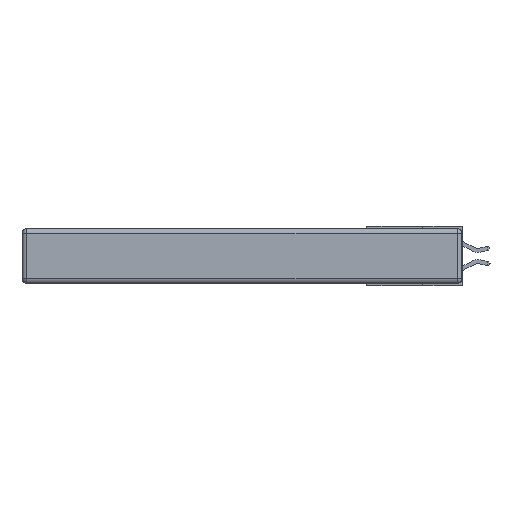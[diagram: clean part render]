
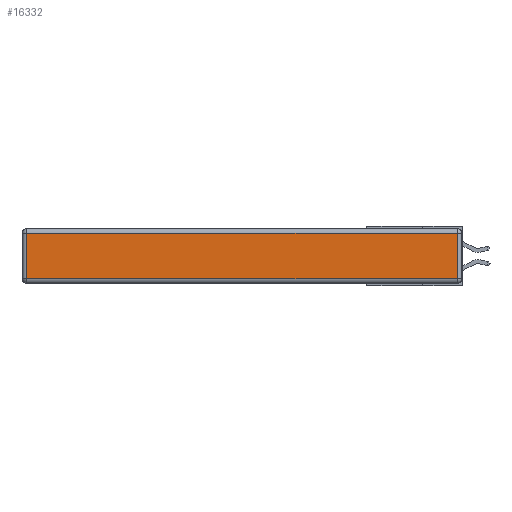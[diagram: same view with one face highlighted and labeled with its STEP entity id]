
A CAD part, left-side view. The second image highlights one B-rep face of the part: STEP entity #16332.
In plain terms, the highlighted planar face has unit normal (-1, 0, 0).
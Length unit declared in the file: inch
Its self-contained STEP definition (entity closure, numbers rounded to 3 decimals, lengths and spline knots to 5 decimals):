
#822 = CARTESIAN_POINT ( 'NONE',  ( 0., 0.03, -0.313 ) ) ;
#1218 = EDGE_CURVE ( 'NONE', #12406, #23030, #22073, .T. ) ;
#3416 = CARTESIAN_POINT ( 'NONE',  ( 0., 2.72, -0.03 ) ) ;
#3849 = EDGE_CURVE ( 'NONE', #23030, #23512, #14712, .T. ) ;
#5129 = CARTESIAN_POINT ( 'NONE',  ( 0., 0.03, -0.343 ) ) ;
#5376 = LINE ( 'NONE', #22428, #11016 ) ;
#5700 = CARTESIAN_POINT ( 'NONE',  ( 0., 0., -0.343 ) ) ;
#7047 = VERTEX_POINT ( 'NONE', #26728 ) ;
#7717 = ORIENTED_EDGE ( 'NONE', *, *, #27499, .T. ) ;
#11016 = VECTOR ( 'NONE', #17418, 39.37008 ) ;
#12406 = VERTEX_POINT ( 'NONE', #3416 ) ;
#13773 = ORIENTED_EDGE ( 'NONE', *, *, #3849, .T. ) ;
#14712 = LINE ( 'NONE', #22365, #24995 ) ;
#14990 = LINE ( 'NONE', #5129, #31386 ) ;
#15614 = VECTOR ( 'NONE', #21941, 39.37008 ) ;
#15996 = EDGE_CURVE ( 'NONE', #7047, #12406, #5376, .T. ) ;
#16332 = ADVANCED_FACE ( 'NONE', ( #17983 ), #20392, .T. ) ;
#16710 = ORIENTED_EDGE ( 'NONE', *, *, #15996, .T. ) ;
#17322 = DIRECTION ( 'NONE',  ( 0., -1., 0. ) ) ;
#17418 = DIRECTION ( 'NONE',  ( 0., 1., 0. ) ) ;
#17586 = DIRECTION ( 'NONE',  ( -1., 0., 0. ) ) ;
#17983 = FACE_OUTER_BOUND ( 'NONE', #28464, .T. ) ;
#20060 = DIRECTION ( 'NONE',  ( 0., 0., 1. ) ) ;
#20392 = PLANE ( 'NONE',  #26870 ) ;
#21864 = ORIENTED_EDGE ( 'NONE', *, *, #1218, .T. ) ;
#21941 = DIRECTION ( 'NONE',  ( 0., 0., -1. ) ) ;
#22073 = LINE ( 'NONE', #31642, #15614 ) ;
#22365 = CARTESIAN_POINT ( 'NONE',  ( 0., 0., -0.313 ) ) ;
#22428 = CARTESIAN_POINT ( 'NONE',  ( 0., 2.75, -0.03 ) ) ;
#23030 = VERTEX_POINT ( 'NONE', #28006 ) ;
#23512 = VERTEX_POINT ( 'NONE', #822 ) ;
#24995 = VECTOR ( 'NONE', #17322, 39.37008 ) ;
#26728 = CARTESIAN_POINT ( 'NONE',  ( 0., 0.03, -0.03 ) ) ;
#26870 = AXIS2_PLACEMENT_3D ( 'NONE', #5700, #17586, #20060 ) ;
#27499 = EDGE_CURVE ( 'NONE', #23512, #7047, #14990, .T. ) ;
#28006 = CARTESIAN_POINT ( 'NONE',  ( 0., 2.72, -0.313 ) ) ;
#28464 = EDGE_LOOP ( 'NONE', ( #13773, #7717, #16710, #21864 ) ) ;
#30139 = DIRECTION ( 'NONE',  ( 0., 0., 1. ) ) ;
#31386 = VECTOR ( 'NONE', #30139, 39.37008 ) ;
#31642 = CARTESIAN_POINT ( 'NONE',  ( 0., 2.72, -0.343 ) ) ;
